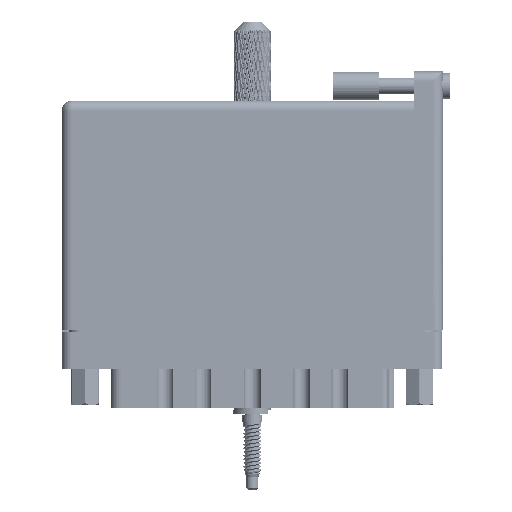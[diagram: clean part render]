
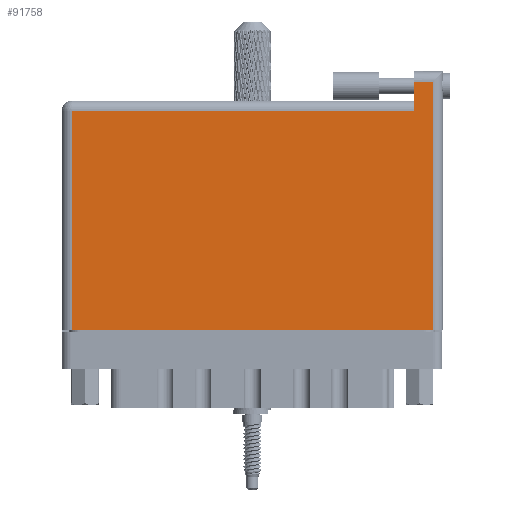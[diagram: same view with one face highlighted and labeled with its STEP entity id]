
A CAD part, front view. The second image highlights one B-rep face of the part: STEP entity #91758.
In plain terms, the highlighted face is planar.
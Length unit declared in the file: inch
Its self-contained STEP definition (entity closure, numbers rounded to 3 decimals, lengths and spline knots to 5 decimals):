
#2506 = VECTOR ( 'NONE', #60181, 39.37008 ) ;
#3311 = EDGE_CURVE ( 'NONE', #73458, #37385, #84683, .T. ) ;
#4483 = CARTESIAN_POINT ( 'NONE',  ( 2.53, 0., 0. ) ) ;
#5940 = DIRECTION ( 'NONE',  ( 0., -1., 0. ) ) ;
#8123 = VECTOR ( 'NONE', #5940, 39.37008 ) ;
#10759 = VECTOR ( 'NONE', #109742, 39.37008 ) ;
#13890 = ORIENTED_EDGE ( 'NONE', *, *, #34014, .T. ) ;
#16939 = CARTESIAN_POINT ( 'NONE',  ( 0.07, 1.496, 0. ) ) ;
#18569 = VERTEX_POINT ( 'NONE', #27737 ) ;
#18615 = EDGE_CURVE ( 'NONE', #18569, #31750, #61899, .T. ) ;
#21240 = VERTEX_POINT ( 'NONE', #76365 ) ;
#22099 = CARTESIAN_POINT ( 'NONE',  ( 0., 1.696, 0. ) ) ;
#23525 = PLANE ( 'NONE',  #66381 ) ;
#24909 = ORIENTED_EDGE ( 'NONE', *, *, #85647, .T. ) ;
#27737 = CARTESIAN_POINT ( 'NONE',  ( 0.07, 0., 0. ) ) ;
#28716 = LINE ( 'NONE', #100713, #2506 ) ;
#29097 = VECTOR ( 'NONE', #91200, 39.37008 ) ;
#31750 = VERTEX_POINT ( 'NONE', #4483 ) ;
#34014 = EDGE_CURVE ( 'NONE', #37385, #18569, #100681, .T. ) ;
#34515 = FACE_OUTER_BOUND ( 'NONE', #52834, .T. ) ;
#36993 = LINE ( 'NONE', #22099, #10759 ) ;
#37385 = VERTEX_POINT ( 'NONE', #16939 ) ;
#39428 = VERTEX_POINT ( 'NONE', #47559 ) ;
#44726 = ORIENTED_EDGE ( 'NONE', *, *, #104931, .T. ) ;
#47559 = CARTESIAN_POINT ( 'NONE',  ( 2.53, 1.696, 0. ) ) ;
#49832 = ORIENTED_EDGE ( 'NONE', *, *, #3311, .T. ) ;
#51978 = VECTOR ( 'NONE', #117701, 39.37008 ) ;
#52834 = EDGE_LOOP ( 'NONE', ( #71772, #121896, #24909, #44726, #49832, #13890 ) ) ;
#60181 = DIRECTION ( 'NONE',  ( 0., 1., 0. ) ) ;
#60428 = VECTOR ( 'NONE', #93189, 39.37008 ) ;
#61899 = LINE ( 'NONE', #73738, #60428 ) ;
#62245 = CARTESIAN_POINT ( 'NONE',  ( 0., 1.496, 0. ) ) ;
#66381 = AXIS2_PLACEMENT_3D ( 'NONE', #83925, #83078, #122728 ) ;
#71772 = ORIENTED_EDGE ( 'NONE', *, *, #18615, .T. ) ;
#73458 = VERTEX_POINT ( 'NONE', #79617 ) ;
#73738 = CARTESIAN_POINT ( 'NONE',  ( 0., 0., 0. ) ) ;
#75210 = EDGE_CURVE ( 'NONE', #31750, #39428, #28716, .T. ) ;
#76365 = CARTESIAN_POINT ( 'NONE',  ( 2.403, 1.696, 0. ) ) ;
#76714 = CARTESIAN_POINT ( 'NONE',  ( 2.403, 1.766, 0. ) ) ;
#76783 = LINE ( 'NONE', #76714, #51978 ) ;
#79617 = CARTESIAN_POINT ( 'NONE',  ( 2.403, 1.496, 0. ) ) ;
#83078 = DIRECTION ( 'NONE',  ( 0., 0., -1. ) ) ;
#83925 = CARTESIAN_POINT ( 'NONE',  ( 0., 1.566, 0. ) ) ;
#84683 = LINE ( 'NONE', #62245, #29097 ) ;
#84879 = CARTESIAN_POINT ( 'NONE',  ( 0.07, 0., 0. ) ) ;
#85647 = EDGE_CURVE ( 'NONE', #39428, #21240, #36993, .T. ) ;
#91200 = DIRECTION ( 'NONE',  ( -1., 0., 0. ) ) ;
#91758 = ADVANCED_FACE ( 'NONE', ( #34515 ), #23525, .F. ) ;
#93189 = DIRECTION ( 'NONE',  ( 1., 0., 0. ) ) ;
#100681 = LINE ( 'NONE', #84879, #8123 ) ;
#100713 = CARTESIAN_POINT ( 'NONE',  ( 2.53, 1.766, 0. ) ) ;
#104931 = EDGE_CURVE ( 'NONE', #21240, #73458, #76783, .T. ) ;
#109742 = DIRECTION ( 'NONE',  ( -1., 0., 0. ) ) ;
#117701 = DIRECTION ( 'NONE',  ( 0., -1., 0. ) ) ;
#121896 = ORIENTED_EDGE ( 'NONE', *, *, #75210, .T. ) ;
#122728 = DIRECTION ( 'NONE',  ( -1., 0., 0. ) ) ;
